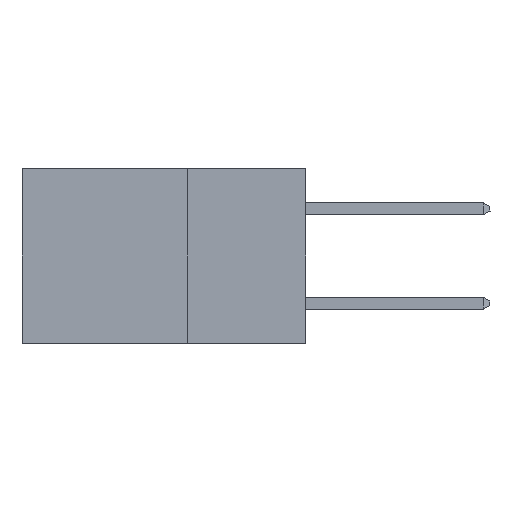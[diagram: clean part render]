
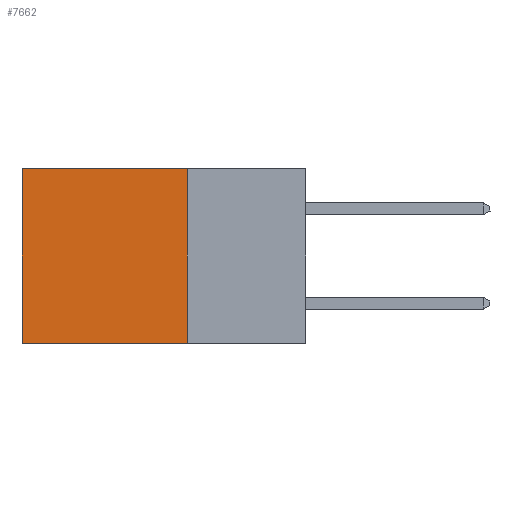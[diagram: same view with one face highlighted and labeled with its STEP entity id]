
A CAD part, left-side view. The second image highlights one B-rep face of the part: STEP entity #7662.
In plain terms, the highlighted planar face has unit normal (-1, 0, 0).
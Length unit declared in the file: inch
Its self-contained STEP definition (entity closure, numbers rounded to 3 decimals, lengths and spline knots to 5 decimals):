
#1044 = EDGE_CURVE ( 'NONE', #26335, #20830, #15351, .T. ) ;
#1337 = EDGE_CURVE ( 'NONE', #18347, #19544, #13684, .T. ) ;
#1726 = VECTOR ( 'NONE', #18959, 39.37008 ) ;
#3867 = DIRECTION ( 'NONE',  ( 1., 0., 0. ) ) ;
#4338 = CARTESIAN_POINT ( 'NONE',  ( 0.298, 0.6, -0.37 ) ) ;
#5581 = EDGE_LOOP ( 'NONE', ( #19703, #11900, #5839, #26942 ) ) ;
#5839 = ORIENTED_EDGE ( 'NONE', *, *, #9631, .F. ) ;
#6046 = CARTESIAN_POINT ( 'NONE',  ( 0.298, 0.25, 0. ) ) ;
#6777 = DIRECTION ( 'NONE',  ( 0., 1., 0. ) ) ;
#7662 = ADVANCED_FACE ( 'NONE', ( #9748 ), #16546, .F. ) ;
#9368 = CARTESIAN_POINT ( 'NONE',  ( 0.298, 0.25, -0.37 ) ) ;
#9631 = EDGE_CURVE ( 'NONE', #26335, #18347, #19961, .T. ) ;
#9748 = FACE_OUTER_BOUND ( 'NONE', #5581, .T. ) ;
#11038 = CARTESIAN_POINT ( 'NONE',  ( 0.298, 0.25, 0. ) ) ;
#11712 = VECTOR ( 'NONE', #22854, 39.37008 ) ;
#11727 = AXIS2_PLACEMENT_3D ( 'NONE', #14467, #3867, #18950 ) ;
#11900 = ORIENTED_EDGE ( 'NONE', *, *, #1337, .F. ) ;
#13411 = CARTESIAN_POINT ( 'NONE',  ( 0.298, 0.6, 0. ) ) ;
#13684 = LINE ( 'NONE', #25216, #1726 ) ;
#14467 = CARTESIAN_POINT ( 'NONE',  ( 0.298, 0.25, 0. ) ) ;
#15351 = LINE ( 'NONE', #11038, #20270 ) ;
#15438 = CARTESIAN_POINT ( 'NONE',  ( 0.298, 0.6, 0. ) ) ;
#15703 = CARTESIAN_POINT ( 'NONE',  ( 0.298, 0.25, 0. ) ) ;
#16546 = PLANE ( 'NONE',  #11727 ) ;
#17446 = DIRECTION ( 'NONE',  ( 0., 0., -1. ) ) ;
#17519 = LINE ( 'NONE', #13411, #20188 ) ;
#18347 = VERTEX_POINT ( 'NONE', #9368 ) ;
#18950 = DIRECTION ( 'NONE',  ( 0., 0., -1. ) ) ;
#18959 = DIRECTION ( 'NONE',  ( 0., 1., 0. ) ) ;
#19544 = VERTEX_POINT ( 'NONE', #4338 ) ;
#19703 = ORIENTED_EDGE ( 'NONE', *, *, #20262, .T. ) ;
#19961 = LINE ( 'NONE', #15703, #11712 ) ;
#20188 = VECTOR ( 'NONE', #17446, 39.37008 ) ;
#20262 = EDGE_CURVE ( 'NONE', #20830, #19544, #17519, .T. ) ;
#20270 = VECTOR ( 'NONE', #6777, 39.37008 ) ;
#20830 = VERTEX_POINT ( 'NONE', #15438 ) ;
#22854 = DIRECTION ( 'NONE',  ( 0., 0., -1. ) ) ;
#25216 = CARTESIAN_POINT ( 'NONE',  ( 0.298, 0.25, -0.37 ) ) ;
#26335 = VERTEX_POINT ( 'NONE', #6046 ) ;
#26942 = ORIENTED_EDGE ( 'NONE', *, *, #1044, .T. ) ;
